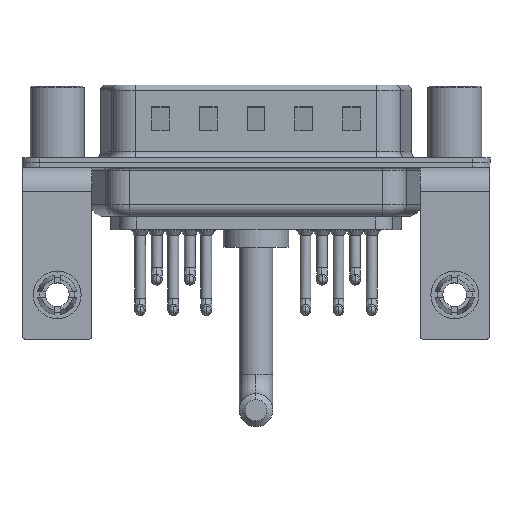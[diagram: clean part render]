
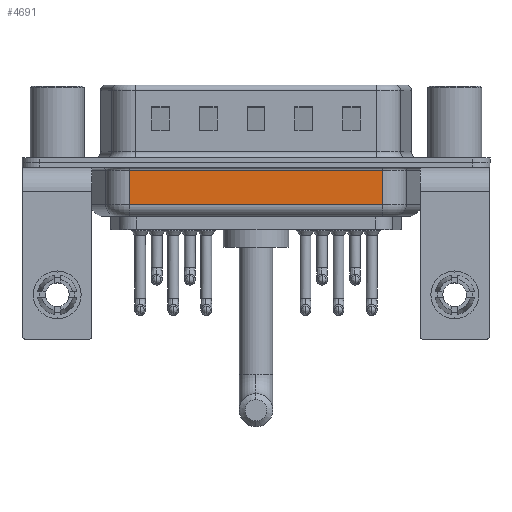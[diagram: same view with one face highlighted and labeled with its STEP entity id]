
A CAD part, front view. The second image highlights one B-rep face of the part: STEP entity #4691.
In plain terms, the highlighted planar face has unit normal (0, -1, 0).
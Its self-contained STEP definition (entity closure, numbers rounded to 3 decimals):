
#513 = VERTEX_POINT ( 'NONE', #1528 ) ;
#1528 = CARTESIAN_POINT ( 'NONE',  ( 27.269, -5.35, -3.5 ) ) ;
#3195 = VERTEX_POINT ( 'NONE', #7047 ) ;
#3434 = LINE ( 'NONE', #23290, #18215 ) ;
#3635 = VECTOR ( 'NONE', #16331, 1000. ) ;
#3936 = CARTESIAN_POINT ( 'NONE',  ( 6.031, -5.35, -3.5 ) ) ;
#4691 = ADVANCED_FACE ( 'NONE', ( #16714 ), #12432, .F. ) ;
#4929 = DIRECTION ( 'NONE',  ( 0., 0., 1. ) ) ;
#7047 = CARTESIAN_POINT ( 'NONE',  ( 6.031, -5.35, -0.65 ) ) ;
#7568 = ORIENTED_EDGE ( 'NONE', *, *, #20918, .F. ) ;
#8116 = CARTESIAN_POINT ( 'NONE',  ( 27.269, -5.35, -0.65 ) ) ;
#12432 = PLANE ( 'NONE',  #17402 ) ;
#12449 = LINE ( 'NONE', #16610, #22393 ) ;
#14058 = VERTEX_POINT ( 'NONE', #15318 ) ;
#14769 = EDGE_LOOP ( 'NONE', ( #7568, #19618, #23472, #21704 ) ) ;
#15318 = CARTESIAN_POINT ( 'NONE',  ( 6.031, -5.35, -3.5 ) ) ;
#15356 = EDGE_CURVE ( 'NONE', #513, #16803, #12449, .T. ) ;
#16331 = DIRECTION ( 'NONE',  ( -1., 0., 0. ) ) ;
#16449 = DIRECTION ( 'NONE',  ( 0., 1., 0. ) ) ;
#16610 = CARTESIAN_POINT ( 'NONE',  ( 27.269, -5.35, -4.5 ) ) ;
#16714 = FACE_OUTER_BOUND ( 'NONE', #14769, .T. ) ;
#16780 = EDGE_CURVE ( 'NONE', #14058, #513, #20052, .T. ) ;
#16803 = VERTEX_POINT ( 'NONE', #8116 ) ;
#17402 = AXIS2_PLACEMENT_3D ( 'NONE', #26493, #16449, #18736 ) ;
#18215 = VECTOR ( 'NONE', #4929, 1000. ) ;
#18736 = DIRECTION ( 'NONE',  ( 0., 0., 1. ) ) ;
#19618 = ORIENTED_EDGE ( 'NONE', *, *, #16780, .T. ) ;
#20052 = LINE ( 'NONE', #3936, #24947 ) ;
#20918 = EDGE_CURVE ( 'NONE', #14058, #3195, #3434, .T. ) ;
#21704 = ORIENTED_EDGE ( 'NONE', *, *, #26119, .T. ) ;
#22241 = CARTESIAN_POINT ( 'NONE',  ( 6.031, -5.35, -0.65 ) ) ;
#22393 = VECTOR ( 'NONE', #24771, 1000. ) ;
#23290 = CARTESIAN_POINT ( 'NONE',  ( 6.031, -5.35, -4.5 ) ) ;
#23472 = ORIENTED_EDGE ( 'NONE', *, *, #15356, .T. ) ;
#24048 = DIRECTION ( 'NONE',  ( 1., 0., 0. ) ) ;
#24771 = DIRECTION ( 'NONE',  ( 0., 0., 1. ) ) ;
#24947 = VECTOR ( 'NONE', #24048, 1000. ) ;
#26119 = EDGE_CURVE ( 'NONE', #16803, #3195, #26507, .T. ) ;
#26493 = CARTESIAN_POINT ( 'NONE',  ( 6.031, -5.35, -4.5 ) ) ;
#26507 = LINE ( 'NONE', #22241, #3635 ) ;
